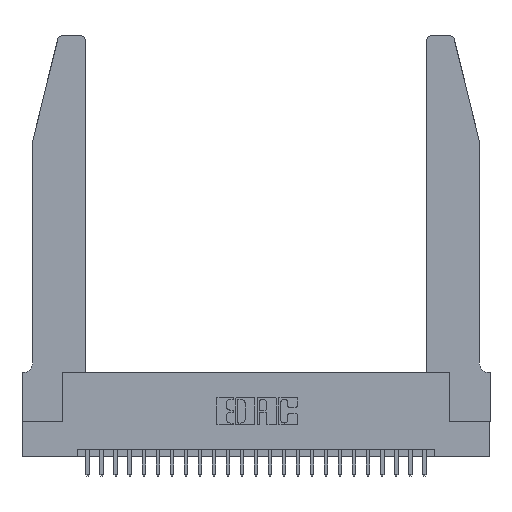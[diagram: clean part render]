
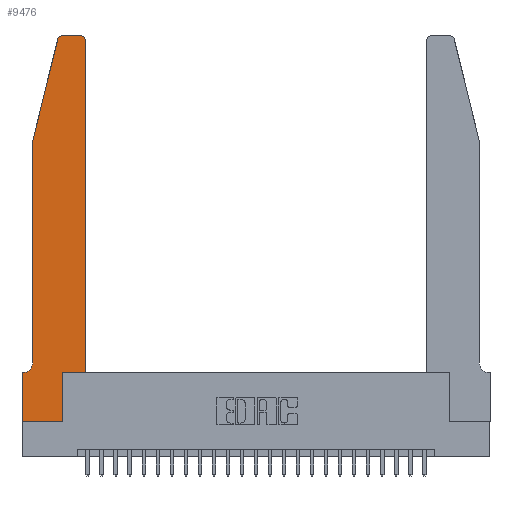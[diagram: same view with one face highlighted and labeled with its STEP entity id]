
A CAD part, top view. The second image highlights one B-rep face of the part: STEP entity #9476.
In plain terms, the highlighted planar face has unit normal (0, 0, 1).
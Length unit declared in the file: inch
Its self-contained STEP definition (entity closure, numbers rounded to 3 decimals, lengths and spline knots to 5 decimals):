
#697 = CIRCLE ( 'NONE', #25119, 0.03 ) ;
#1037 = LINE ( 'NONE', #13704, #6011 ) ;
#1326 = CARTESIAN_POINT ( 'NONE',  ( 0.2865, 0., 0.37 ) ) ;
#1333 = AXIS2_PLACEMENT_3D ( 'NONE', #16625, #4349, #18695 ) ;
#1337 = CARTESIAN_POINT ( 'NONE',  ( 0.0755, 0.42, 0.37 ) ) ;
#1511 = FACE_OUTER_BOUND ( 'NONE', #9733, .T. ) ;
#1645 = EDGE_CURVE ( 'NONE', #21758, #23755, #1037, .T. ) ;
#1748 = DIRECTION ( 'NONE',  ( 0., 1., 0. ) ) ;
#2077 = CARTESIAN_POINT ( 'NONE',  ( 0., 0., 0.37 ) ) ;
#2134 = DIRECTION ( 'NONE',  ( 0., -1., 0. ) ) ;
#2183 = LINE ( 'NONE', #24870, #17328 ) ;
#2252 = LINE ( 'NONE', #20687, #13900 ) ;
#2404 = VECTOR ( 'NONE', #15611, 39.37008 ) ;
#3097 = ORIENTED_EDGE ( 'NONE', *, *, #23531, .T. ) ;
#3189 = VERTEX_POINT ( 'NONE', #21310 ) ;
#4349 = DIRECTION ( 'NONE',  ( 0., 0., 1. ) ) ;
#4574 = AXIS2_PLACEMENT_3D ( 'NONE', #17305, #5040, #19352 ) ;
#4756 = VERTEX_POINT ( 'NONE', #1326 ) ;
#4913 = AXIS2_PLACEMENT_3D ( 'NONE', #8744, #22994, #10786 ) ;
#5040 = DIRECTION ( 'NONE',  ( 0., 0., -1. ) ) ;
#5542 = CARTESIAN_POINT ( 'NONE',  ( 0.25487, 2.72718, 0.37 ) ) ;
#5708 = ORIENTED_EDGE ( 'NONE', *, *, #25497, .T. ) ;
#5951 = CARTESIAN_POINT ( 'NONE',  ( 0.284, 2.72, 0.37 ) ) ;
#5968 = CARTESIAN_POINT ( 'NONE',  ( 0.0755, 2., 0.37 ) ) ;
#6011 = VECTOR ( 'NONE', #1748, 39.37008 ) ;
#6240 = VERTEX_POINT ( 'NONE', #14759 ) ;
#6703 = LINE ( 'NONE', #25777, #2404 ) ;
#6798 = CARTESIAN_POINT ( 'NONE',  ( 0.4505, 0.35, 0.37 ) ) ;
#6864 = VECTOR ( 'NONE', #19513, 39.37008 ) ;
#7023 = ORIENTED_EDGE ( 'NONE', *, *, #8034, .T. ) ;
#7061 = CARTESIAN_POINT ( 'NONE',  ( 0.2605, 2.75, 0.37 ) ) ;
#7103 = CARTESIAN_POINT ( 'NONE',  ( 0.2865, 0.35, 0.37 ) ) ;
#7104 = VERTEX_POINT ( 'NONE', #1337 ) ;
#7294 = CARTESIAN_POINT ( 'NONE',  ( 0.0755, 2., 0.37 ) ) ;
#7360 = ORIENTED_EDGE ( 'NONE', *, *, #13435, .T. ) ;
#8034 = EDGE_CURVE ( 'NONE', #14393, #7104, #2252, .T. ) ;
#8051 = DIRECTION ( 'NONE',  ( 1., 0., 0. ) ) ;
#8353 = DIRECTION ( 'NONE',  ( -1., 0., 0. ) ) ;
#8744 = CARTESIAN_POINT ( 'NONE',  ( 0.4205, 2.72, 0.37 ) ) ;
#9012 = VERTEX_POINT ( 'NONE', #7103 ) ;
#9476 = ADVANCED_FACE ( 'NONE', ( #1511 ), #22710, .T. ) ;
#9733 = EDGE_LOOP ( 'NONE', ( #22990, #5708, #17238, #7023, #10247, #7360, #10593, #11857, #11555, #3097, #19535, #10962 ) ) ;
#10247 = ORIENTED_EDGE ( 'NONE', *, *, #13737, .T. ) ;
#10593 = ORIENTED_EDGE ( 'NONE', *, *, #23661, .T. ) ;
#10786 = DIRECTION ( 'NONE',  ( 1., 0., 0. ) ) ;
#10792 = EDGE_CURVE ( 'NONE', #23755, #15688, #20471, .T. ) ;
#10962 = ORIENTED_EDGE ( 'NONE', *, *, #10792, .T. ) ;
#11178 = EDGE_CURVE ( 'NONE', #4756, #9012, #6703, .T. ) ;
#11555 = ORIENTED_EDGE ( 'NONE', *, *, #11178, .T. ) ;
#11640 = LINE ( 'NONE', #24267, #26587 ) ;
#11857 = ORIENTED_EDGE ( 'NONE', *, *, #12182, .T. ) ;
#12182 = EDGE_CURVE ( 'NONE', #26060, #4756, #2183, .T. ) ;
#13431 = CIRCLE ( 'NONE', #4574, 0.07 ) ;
#13435 = EDGE_CURVE ( 'NONE', #3189, #6240, #25836, .T. ) ;
#13704 = CARTESIAN_POINT ( 'NONE',  ( 0.4505, 0.35, 0.37 ) ) ;
#13737 = EDGE_CURVE ( 'NONE', #7104, #3189, #13431, .T. ) ;
#13900 = VECTOR ( 'NONE', #2134, 39.37008 ) ;
#14393 = VERTEX_POINT ( 'NONE', #5968 ) ;
#14759 = CARTESIAN_POINT ( 'NONE',  ( 0., 0.35, 0.37 ) ) ;
#15110 = CARTESIAN_POINT ( 'NONE',  ( 0.284, 2.75, 0.37 ) ) ;
#15611 = DIRECTION ( 'NONE',  ( 0., 1., 0. ) ) ;
#15688 = VERTEX_POINT ( 'NONE', #18521 ) ;
#16625 = CARTESIAN_POINT ( 'NONE',  ( 0., 0.35, 0.37 ) ) ;
#16903 = VECTOR ( 'NONE', #17318, 39.37008 ) ;
#17071 = LINE ( 'NONE', #7294, #6864 ) ;
#17238 = ORIENTED_EDGE ( 'NONE', *, *, #17443, .T. ) ;
#17305 = CARTESIAN_POINT ( 'NONE',  ( 0.0055, 0.42, 0.37 ) ) ;
#17318 = DIRECTION ( 'NONE',  ( -1., 0., 0. ) ) ;
#17328 = VECTOR ( 'NONE', #22841, 39.37008 ) ;
#17443 = EDGE_CURVE ( 'NONE', #26673, #14393, #17071, .T. ) ;
#17544 = LINE ( 'NONE', #7061, #16903 ) ;
#18521 = CARTESIAN_POINT ( 'NONE',  ( 0.4205, 2.75, 0.37 ) ) ;
#18648 = LINE ( 'NONE', #2077, #23417 ) ;
#18695 = DIRECTION ( 'NONE',  ( 1., 0., 0. ) ) ;
#19352 = DIRECTION ( 'NONE',  ( -1., 0., 0. ) ) ;
#19513 = DIRECTION ( 'NONE',  ( -0.239, -0.971, 0. ) ) ;
#19535 = ORIENTED_EDGE ( 'NONE', *, *, #1645, .T. ) ;
#20254 = DIRECTION ( 'NONE',  ( 0., 0., 1. ) ) ;
#20471 = CIRCLE ( 'NONE', #4913, 0.03 ) ;
#20472 = VECTOR ( 'NONE', #8353, 39.37008 ) ;
#20687 = CARTESIAN_POINT ( 'NONE',  ( 0.0755, 2., 0.37 ) ) ;
#21310 = CARTESIAN_POINT ( 'NONE',  ( 0.0055, 0.35, 0.37 ) ) ;
#21758 = VERTEX_POINT ( 'NONE', #6798 ) ;
#22710 = PLANE ( 'NONE',  #1333 ) ;
#22841 = DIRECTION ( 'NONE',  ( 1., 0., 0. ) ) ;
#22990 = ORIENTED_EDGE ( 'NONE', *, *, #25243, .T. ) ;
#22994 = DIRECTION ( 'NONE',  ( 0., 0., 1. ) ) ;
#23417 = VECTOR ( 'NONE', #24623, 39.37008 ) ;
#23531 = EDGE_CURVE ( 'NONE', #9012, #21758, #11640, .T. ) ;
#23661 = EDGE_CURVE ( 'NONE', #6240, #26060, #18648, .T. ) ;
#23755 = VERTEX_POINT ( 'NONE', #24880 ) ;
#24187 = DIRECTION ( 'NONE',  ( 1., 0., 0. ) ) ;
#24267 = CARTESIAN_POINT ( 'NONE',  ( 0.4505, 0.35, 0.37 ) ) ;
#24532 = VERTEX_POINT ( 'NONE', #15110 ) ;
#24623 = DIRECTION ( 'NONE',  ( 0., -1., 0. ) ) ;
#24870 = CARTESIAN_POINT ( 'NONE',  ( 0., 0., 0.37 ) ) ;
#24880 = CARTESIAN_POINT ( 'NONE',  ( 0.4505, 2.72, 0.37 ) ) ;
#25119 = AXIS2_PLACEMENT_3D ( 'NONE', #5951, #20254, #8051 ) ;
#25243 = EDGE_CURVE ( 'NONE', #15688, #24532, #17544, .T. ) ;
#25497 = EDGE_CURVE ( 'NONE', #24532, #26673, #697, .T. ) ;
#25777 = CARTESIAN_POINT ( 'NONE',  ( 0.2865, 0.35, 0.37 ) ) ;
#25825 = CARTESIAN_POINT ( 'NONE',  ( 0., 0., 0.37 ) ) ;
#25836 = LINE ( 'NONE', #26573, #20472 ) ;
#26060 = VERTEX_POINT ( 'NONE', #25825 ) ;
#26573 = CARTESIAN_POINT ( 'NONE',  ( 0.0755, 0.35, 0.37 ) ) ;
#26587 = VECTOR ( 'NONE', #24187, 39.37008 ) ;
#26673 = VERTEX_POINT ( 'NONE', #5542 ) ;
